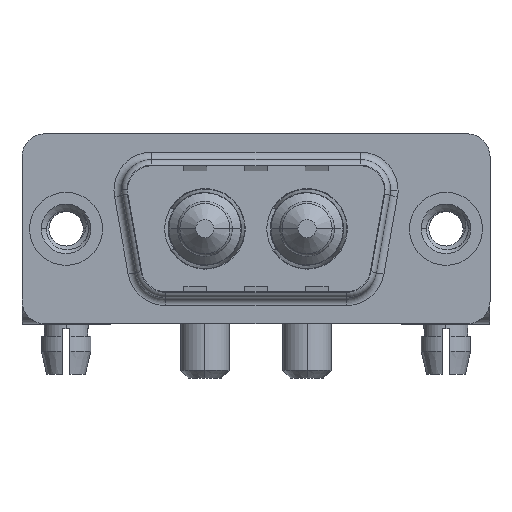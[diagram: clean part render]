
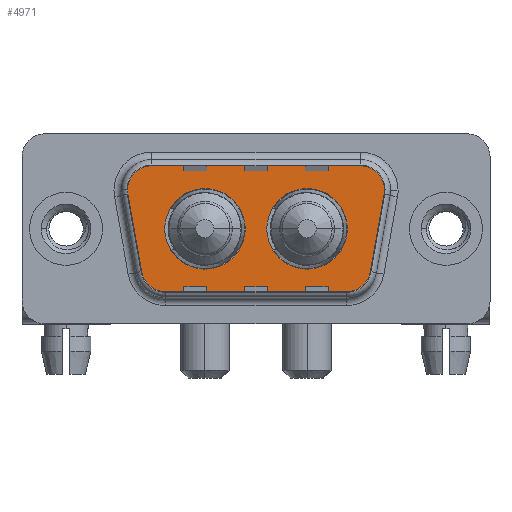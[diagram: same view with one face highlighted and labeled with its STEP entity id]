
A CAD part, top view. The second image highlights one B-rep face of the part: STEP entity #4971.
In plain terms, the highlighted planar face has unit normal (0, 0, 1).
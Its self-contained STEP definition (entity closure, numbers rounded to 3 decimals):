
#130 = CIRCLE ( 'NONE', #2368, 2. ) ;
#175 = VERTEX_POINT ( 'NONE', #6731 ) ;
#279 = CARTESIAN_POINT ( 'NONE',  ( 9.14, 0., 0. ) ) ;
#429 = DIRECTION ( 'NONE',  ( 0., 0., 1. ) ) ;
#504 = CARTESIAN_POINT ( 'NONE',  ( 19.564, 2.9, 0. ) ) ;
#509 = EDGE_CURVE ( 'NONE', #13867, #12634, #10368, .T. ) ;
#737 = CARTESIAN_POINT ( 'NONE',  ( 21.534, 2.553, 0. ) ) ;
#858 = DIRECTION ( 'NONE',  ( 0., 0., 1. ) ) ;
#991 = CARTESIAN_POINT ( 'NONE',  ( 9.14, 0., 0. ) ) ;
#1219 = AXIS2_PLACEMENT_3D ( 'NONE', #4903, #5881, #5212 ) ;
#1323 = VERTEX_POINT ( 'NONE', #4127 ) ;
#1525 = LINE ( 'NONE', #2374, #6016 ) ;
#1636 = CARTESIAN_POINT ( 'NONE',  ( 5.436, 4.9, 0. ) ) ;
#1916 = PLANE ( 'NONE',  #4059 ) ;
#2364 = EDGE_CURVE ( 'NONE', #7351, #5394, #5282, .T. ) ;
#2368 = AXIS2_PLACEMENT_3D ( 'NONE', #8811, #3463, #7759 ) ;
#2374 = CARTESIAN_POINT ( 'NONE',  ( 3.466, 2.553, 0. ) ) ;
#2397 = EDGE_CURVE ( 'NONE', #8982, #11069, #13435, .T. ) ;
#2466 = DIRECTION ( 'NONE',  ( 1., 0., 0. ) ) ;
#2578 = VECTOR ( 'NONE', #13319, 1000. ) ;
#2592 = DIRECTION ( 'NONE',  ( 0.174, -0.985, 0. ) ) ;
#2844 = CARTESIAN_POINT ( 'NONE',  ( 6.459, -2.9, 0. ) ) ;
#3138 = DIRECTION ( 'NONE',  ( 0., 0., 1. ) ) ;
#3268 = AXIS2_PLACEMENT_3D ( 'NONE', #279, #429, #2466 ) ;
#3463 = DIRECTION ( 'NONE',  ( 0., 0., 1. ) ) ;
#3745 = AXIS2_PLACEMENT_3D ( 'NONE', #504, #10147, #5712 ) ;
#3757 = CARTESIAN_POINT ( 'NONE',  ( 18.51, 0., 0. ) ) ;
#3831 = DIRECTION ( 'NONE',  ( 0., 0., 1. ) ) ;
#4059 = AXIS2_PLACEMENT_3D ( 'NONE', #11368, #858, #10306 ) ;
#4094 = DIRECTION ( 'NONE',  ( 1., 0., 0. ) ) ;
#4127 = CARTESIAN_POINT ( 'NONE',  ( 20.511, -3.247, 0. ) ) ;
#4374 = CIRCLE ( 'NONE', #1219, 2.65 ) ;
#4522 = ORIENTED_EDGE ( 'NONE', *, *, #12558, .T. ) ;
#4631 = ORIENTED_EDGE ( 'NONE', *, *, #8003, .F. ) ;
#4646 = DIRECTION ( 'NONE',  ( 1., 0., 0. ) ) ;
#4696 = ORIENTED_EDGE ( 'NONE', *, *, #13320, .T. ) ;
#4701 = ORIENTED_EDGE ( 'NONE', *, *, #10934, .T. ) ;
#4903 = CARTESIAN_POINT ( 'NONE',  ( 15.86, 0., 0. ) ) ;
#4971 = ADVANCED_FACE ( 'NONE', ( #8337, #13778, #8132 ), #1916, .T. ) ;
#5035 = CARTESIAN_POINT ( 'NONE',  ( 19.564, 4.9, 0. ) ) ;
#5143 = DIRECTION ( 'NONE',  ( 1., 0., 0. ) ) ;
#5212 = DIRECTION ( 'NONE',  ( 1., 0., 0. ) ) ;
#5282 = CIRCLE ( 'NONE', #13199, 2.65 ) ;
#5287 = DIRECTION ( 'NONE',  ( 0., 0., 1. ) ) ;
#5394 = VERTEX_POINT ( 'NONE', #3757 ) ;
#5515 = CIRCLE ( 'NONE', #3268, 2.65 ) ;
#5712 = DIRECTION ( 'NONE',  ( -1., 0., 0. ) ) ;
#5785 = DIRECTION ( 'NONE',  ( 0., 0., 1. ) ) ;
#5844 = ORIENTED_EDGE ( 'NONE', *, *, #13396, .T. ) ;
#5881 = DIRECTION ( 'NONE',  ( 0., 0., 1. ) ) ;
#5960 = CIRCLE ( 'NONE', #3745, 2. ) ;
#6016 = VECTOR ( 'NONE', #2592, 1000. ) ;
#6405 = EDGE_LOOP ( 'NONE', ( #13410, #12230, #4701, #10097, #9355, #8998, #5844, #4522, #4696 ) ) ;
#6541 = VERTEX_POINT ( 'NONE', #5035 ) ;
#6613 = CARTESIAN_POINT ( 'NONE',  ( 15.86, 0., 0. ) ) ;
#6625 = EDGE_CURVE ( 'NONE', #12070, #1323, #7029, .T. ) ;
#6669 = CARTESIAN_POINT ( 'NONE',  ( 5.436, 4.9, 0. ) ) ;
#6713 = VECTOR ( 'NONE', #4646, 1000. ) ;
#6731 = CARTESIAN_POINT ( 'NONE',  ( 4.489, -3.247, 0. ) ) ;
#6756 = CARTESIAN_POINT ( 'NONE',  ( 21.564, 2.9, 0. ) ) ;
#6795 = ORIENTED_EDGE ( 'NONE', *, *, #8797, .F. ) ;
#6810 = AXIS2_PLACEMENT_3D ( 'NONE', #11657, #3138, #9460 ) ;
#6902 = VECTOR ( 'NONE', #12589, 1000. ) ;
#7029 = CIRCLE ( 'NONE', #6810, 2. ) ;
#7351 = VERTEX_POINT ( 'NONE', #13332 ) ;
#7472 = ORIENTED_EDGE ( 'NONE', *, *, #2397, .F. ) ;
#7475 = EDGE_LOOP ( 'NONE', ( #4631, #10086 ) ) ;
#7523 = CARTESIAN_POINT ( 'NONE',  ( 3.466, 2.553, 0. ) ) ;
#7759 = DIRECTION ( 'NONE',  ( -1., 0., 0. ) ) ;
#7872 = LINE ( 'NONE', #11239, #6713 ) ;
#8003 = EDGE_CURVE ( 'NONE', #5394, #7351, #4374, .T. ) ;
#8041 = DIRECTION ( 'NONE',  ( 1., 0., 0. ) ) ;
#8059 = DIRECTION ( 'NONE',  ( -1., 0., 0. ) ) ;
#8132 = FACE_OUTER_BOUND ( 'NONE', #6405, .T. ) ;
#8337 = FACE_BOUND ( 'NONE', #7475, .T. ) ;
#8356 = AXIS2_PLACEMENT_3D ( 'NONE', #10003, #5785, #8041 ) ;
#8711 = CIRCLE ( 'NONE', #11632, 2. ) ;
#8797 = EDGE_CURVE ( 'NONE', #11069, #8982, #5515, .T. ) ;
#8811 = CARTESIAN_POINT ( 'NONE',  ( 19.564, 2.9, 0. ) ) ;
#8982 = VERTEX_POINT ( 'NONE', #11325 ) ;
#8998 = ORIENTED_EDGE ( 'NONE', *, *, #509, .T. ) ;
#9355 = ORIENTED_EDGE ( 'NONE', *, *, #9391, .T. ) ;
#9385 = LINE ( 'NONE', #737, #6902 ) ;
#9391 = EDGE_CURVE ( 'NONE', #6541, #13867, #10053, .T. ) ;
#9460 = DIRECTION ( 'NONE',  ( 1., 0., 0. ) ) ;
#10003 = CARTESIAN_POINT ( 'NONE',  ( 5.436, 2.9, 0. ) ) ;
#10053 = LINE ( 'NONE', #6669, #2578 ) ;
#10086 = ORIENTED_EDGE ( 'NONE', *, *, #2364, .F. ) ;
#10097 = ORIENTED_EDGE ( 'NONE', *, *, #10852, .T. ) ;
#10147 = DIRECTION ( 'NONE',  ( 0., 0., 1. ) ) ;
#10195 = CARTESIAN_POINT ( 'NONE',  ( 21.534, 2.553, 0. ) ) ;
#10306 = DIRECTION ( 'NONE',  ( 1., 0., 0. ) ) ;
#10313 = CARTESIAN_POINT ( 'NONE',  ( 18.541, -4.9, 0. ) ) ;
#10368 = CIRCLE ( 'NONE', #8356, 2. ) ;
#10536 = CARTESIAN_POINT ( 'NONE',  ( 11.79, 0., 0. ) ) ;
#10777 = EDGE_LOOP ( 'NONE', ( #6795, #7472 ) ) ;
#10783 = CARTESIAN_POINT ( 'NONE',  ( 6.459, -4.9, 0. ) ) ;
#10852 = EDGE_CURVE ( 'NONE', #12855, #6541, #130, .T. ) ;
#10934 = EDGE_CURVE ( 'NONE', #11401, #12855, #5960, .T. ) ;
#10968 = DIRECTION ( 'NONE',  ( 0., 0., 1. ) ) ;
#11069 = VERTEX_POINT ( 'NONE', #10536 ) ;
#11155 = AXIS2_PLACEMENT_3D ( 'NONE', #991, #5287, #4094 ) ;
#11239 = CARTESIAN_POINT ( 'NONE',  ( 6.459, -4.9, 0. ) ) ;
#11325 = CARTESIAN_POINT ( 'NONE',  ( 6.49, 0., 0. ) ) ;
#11368 = CARTESIAN_POINT ( 'NONE',  ( 18.541, -2.9, 0. ) ) ;
#11401 = VERTEX_POINT ( 'NONE', #10195 ) ;
#11632 = AXIS2_PLACEMENT_3D ( 'NONE', #2844, #3831, #8059 ) ;
#11657 = CARTESIAN_POINT ( 'NONE',  ( 18.541, -2.9, 0. ) ) ;
#11971 = EDGE_CURVE ( 'NONE', #1323, #11401, #9385, .T. ) ;
#12070 = VERTEX_POINT ( 'NONE', #10313 ) ;
#12230 = ORIENTED_EDGE ( 'NONE', *, *, #11971, .T. ) ;
#12558 = EDGE_CURVE ( 'NONE', #175, #13601, #8711, .T. ) ;
#12589 = DIRECTION ( 'NONE',  ( 0.174, 0.985, 0. ) ) ;
#12634 = VERTEX_POINT ( 'NONE', #7523 ) ;
#12855 = VERTEX_POINT ( 'NONE', #6756 ) ;
#13199 = AXIS2_PLACEMENT_3D ( 'NONE', #6613, #10968, #5143 ) ;
#13319 = DIRECTION ( 'NONE',  ( -1., 0., 0. ) ) ;
#13320 = EDGE_CURVE ( 'NONE', #13601, #12070, #7872, .T. ) ;
#13332 = CARTESIAN_POINT ( 'NONE',  ( 13.21, 0., 0. ) ) ;
#13396 = EDGE_CURVE ( 'NONE', #12634, #175, #1525, .T. ) ;
#13410 = ORIENTED_EDGE ( 'NONE', *, *, #6625, .T. ) ;
#13435 = CIRCLE ( 'NONE', #11155, 2.65 ) ;
#13601 = VERTEX_POINT ( 'NONE', #10783 ) ;
#13778 = FACE_BOUND ( 'NONE', #10777, .T. ) ;
#13867 = VERTEX_POINT ( 'NONE', #1636 ) ;
